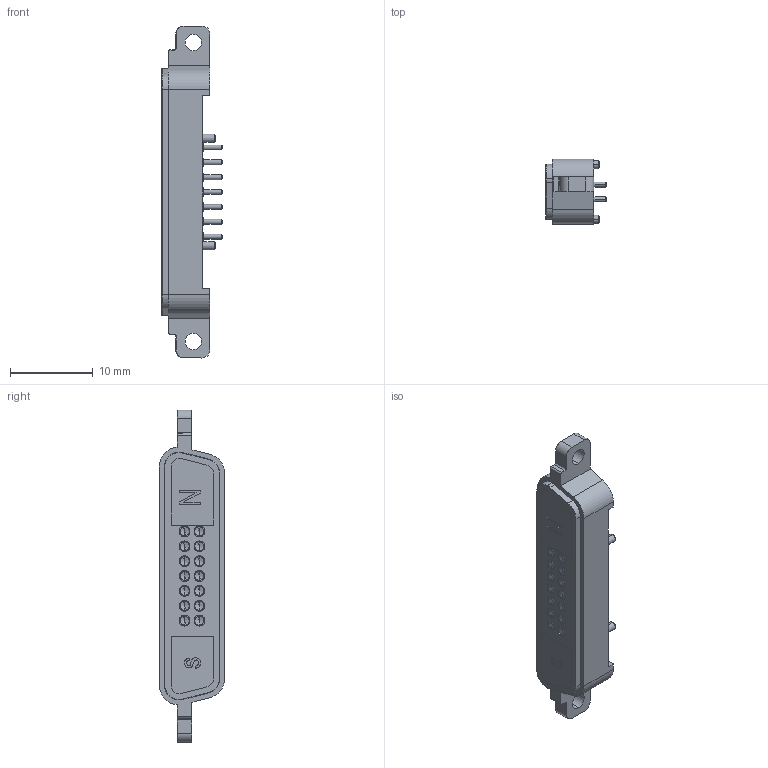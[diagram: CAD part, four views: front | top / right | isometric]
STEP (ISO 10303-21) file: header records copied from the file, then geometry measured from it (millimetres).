
FILE_DESCRIPTION (( 'STEP AP203' ), '1' );
FILE_NAME ('686B1421260123E.STEP', '2023-03-03T12:20:26', ( 'Magnum' ), ( '' ), 'SwSTEP 2.0', 'SolidWorks 2020', '' );
FILE_SCHEMA (( 'CONFIG_CONTROL_DESIGN' ));
Length unit declared in the file: millimetre
Products named in the file (1): 686B1421260123E
Bounding box: 7.35 x 7.9 x 40.2 mm (x, y, z)
Volume: 1235.9 mm3; surface area: 1154.3 mm2
Topology: 1 solids, 1 shells, 431 faces, 980 edges, 597 vertices
Faces by surface type: cylinder 165, plane 120, cone 118, bspline 14, torus 10, sphere 4
Entity records: 12700 total; most frequent: CARTESIAN_POINT 2894, DIRECTION 2155, ORIENTED_EDGE 1896, EDGE_CURVE 948, AXIS2_PLACEMENT_3D 862, VERTEX_POINT 597, EDGE_LOOP 513, CIRCLE 444
